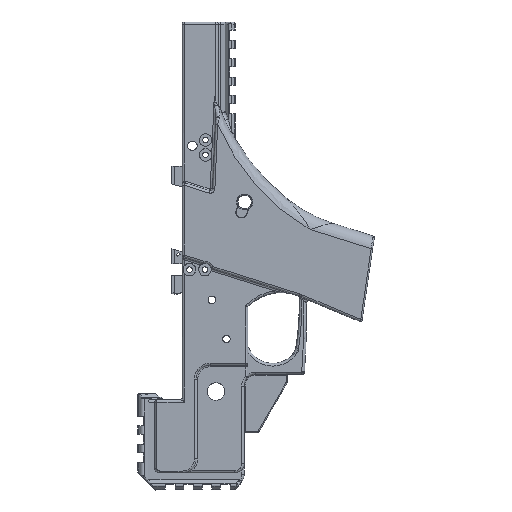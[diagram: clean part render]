
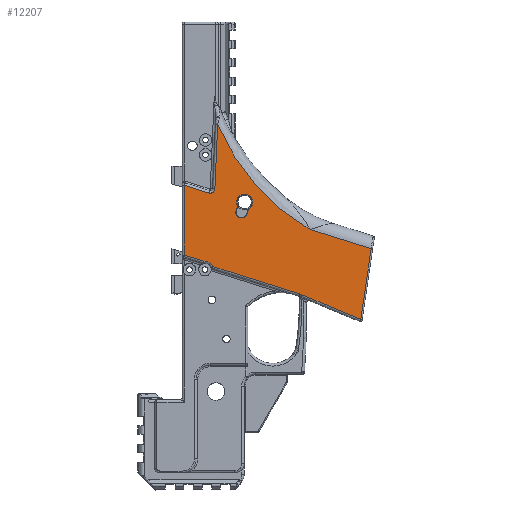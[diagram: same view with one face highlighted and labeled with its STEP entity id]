
A CAD part, left-side view. The second image highlights one B-rep face of the part: STEP entity #12207.
In plain terms, the highlighted planar face has unit normal (-1, 0, 0).
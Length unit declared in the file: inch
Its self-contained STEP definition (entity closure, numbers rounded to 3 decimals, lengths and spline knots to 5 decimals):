
#533=FACE_BOUND('',#3957,.T.);
#667=PLANE('',#13263);
#1186=LINE('',#20847,#2080);
#1207=LINE('',#21066,#2101);
#1209=LINE('',#21087,#2103);
#1211=LINE('',#21092,#2105);
#1212=LINE('',#21096,#2106);
#1213=LINE('',#21098,#2107);
#1214=LINE('',#21100,#2108);
#1215=LINE('',#21104,#2109);
#1216=LINE('',#21108,#2110);
#1217=LINE('',#21112,#2111);
#2080=VECTOR('',#15531,0.3937);
#2101=VECTOR('',#15582,0.3937);
#2103=VECTOR('',#15588,0.3937);
#2105=VECTOR('',#15594,0.3937);
#2106=VECTOR('',#15597,0.3937);
#2107=VECTOR('',#15598,0.3937);
#2108=VECTOR('',#15599,0.3937);
#2109=VECTOR('',#15602,0.3937);
#2110=VECTOR('',#15605,0.3937);
#2111=VECTOR('',#15608,0.3937);
#3211=FACE_OUTER_BOUND('',#3956,.T.);
#3956=EDGE_LOOP('',(#9567,#9568,#9569,#9570,#9571,#9572,#9573,#9574,#9575,
#9576,#9577,#9578));
#3957=EDGE_LOOP('',(#9579,#9580,#9581,#9582));
#4623=CIRCLE('',#13041,4.82183);
#4734=CIRCLE('',#13264,0.1);
#4735=CIRCLE('',#13265,0.1845);
#4736=CIRCLE('',#13266,0.55);
#4737=CIRCLE('',#13267,0.124);
#4738=CIRCLE('',#13268,0.1725);
#5377=VERTEX_POINT('',#19452);
#5378=VERTEX_POINT('',#19458);
#5590=VERTEX_POINT('',#20837);
#5592=VERTEX_POINT('',#20843);
#5626=VERTEX_POINT('',#21065);
#5628=VERTEX_POINT('',#21091);
#5629=VERTEX_POINT('',#21093);
#5630=VERTEX_POINT('',#21095);
#5631=VERTEX_POINT('',#21097);
#5632=VERTEX_POINT('',#21099);
#5633=VERTEX_POINT('',#21101);
#5634=VERTEX_POINT('',#21103);
#5635=VERTEX_POINT('',#21106);
#5636=VERTEX_POINT('',#21107);
#5637=VERTEX_POINT('',#21109);
#5638=VERTEX_POINT('',#21111);
#6702=EDGE_CURVE('',#5378,#5377,#4623,.T.);
#7018=EDGE_CURVE('',#5590,#5592,#1186,.T.);
#7057=EDGE_CURVE('',#5592,#5626,#1207,.T.);
#7061=EDGE_CURVE('',#5378,#5590,#1209,.T.);
#7063=EDGE_CURVE('',#5628,#5377,#1211,.T.);
#7064=EDGE_CURVE('',#5629,#5628,#4734,.T.);
#7065=EDGE_CURVE('',#5630,#5629,#1212,.T.);
#7066=EDGE_CURVE('',#5631,#5630,#1213,.T.);
#7067=EDGE_CURVE('',#5632,#5631,#1214,.T.);
#7068=EDGE_CURVE('',#5633,#5632,#4735,.T.);
#7069=EDGE_CURVE('',#5634,#5633,#1215,.T.);
#7070=EDGE_CURVE('',#5626,#5634,#4736,.T.);
#7071=EDGE_CURVE('',#5635,#5636,#1216,.T.);
#7072=EDGE_CURVE('',#5637,#5635,#4737,.T.);
#7073=EDGE_CURVE('',#5638,#5637,#1217,.T.);
#7074=EDGE_CURVE('',#5636,#5638,#4738,.T.);
#9567=ORIENTED_EDGE('',*,*,#7018,.F.);
#9568=ORIENTED_EDGE('',*,*,#7061,.F.);
#9569=ORIENTED_EDGE('',*,*,#6702,.T.);
#9570=ORIENTED_EDGE('',*,*,#7063,.F.);
#9571=ORIENTED_EDGE('',*,*,#7064,.F.);
#9572=ORIENTED_EDGE('',*,*,#7065,.F.);
#9573=ORIENTED_EDGE('',*,*,#7066,.F.);
#9574=ORIENTED_EDGE('',*,*,#7067,.F.);
#9575=ORIENTED_EDGE('',*,*,#7068,.F.);
#9576=ORIENTED_EDGE('',*,*,#7069,.F.);
#9577=ORIENTED_EDGE('',*,*,#7070,.F.);
#9578=ORIENTED_EDGE('',*,*,#7057,.F.);
#9579=ORIENTED_EDGE('',*,*,#7071,.F.);
#9580=ORIENTED_EDGE('',*,*,#7072,.F.);
#9581=ORIENTED_EDGE('',*,*,#7073,.F.);
#9582=ORIENTED_EDGE('',*,*,#7074,.F.);
#12207=ADVANCED_FACE('',(#3211,#533),#667,.T.);
#13041=AXIS2_PLACEMENT_3D('',#19459,#14977,#14978);
#13263=AXIS2_PLACEMENT_3D('',#21090,#15592,#15593);
#13264=AXIS2_PLACEMENT_3D('',#21094,#15595,#15596);
#13265=AXIS2_PLACEMENT_3D('',#21102,#15600,#15601);
#13266=AXIS2_PLACEMENT_3D('',#21105,#15603,#15604);
#13267=AXIS2_PLACEMENT_3D('',#21110,#15606,#15607);
#13268=AXIS2_PLACEMENT_3D('',#21113,#15609,#15610);
#14977=DIRECTION('center_axis',(1.,0.,0.));
#14978=DIRECTION('ref_axis',(0.,-0.858,0.513));
#15531=DIRECTION('',(0.,0.146,-0.989));
#15582=DIRECTION('',(0.,0.922,0.386));
#15588=DIRECTION('',(0.,-0.954,-0.301));
#15592=DIRECTION('center_axis',(-1.,0.,0.));
#15593=DIRECTION('ref_axis',(0.,0.301,-0.954));
#15594=DIRECTION('',(0.,-0.044,0.999));
#15595=DIRECTION('center_axis',(-1.,0.,0.));
#15596=DIRECTION('ref_axis',(0.,-0.574,-0.819));
#15597=DIRECTION('',(0.,-0.954,-0.301));
#15598=DIRECTION('',(0.,0.,1.));
#15599=DIRECTION('',(0.,0.954,0.301));
#15600=DIRECTION('center_axis',(-1.,0.,0.));
#15601=DIRECTION('ref_axis',(0.,-0.536,0.844));
#15602=DIRECTION('',(0.,0.954,0.301));
#15603=DIRECTION('center_axis',(-1.,0.,0.));
#15604=DIRECTION('ref_axis',(0.,-0.344,0.939));
#15605=DIRECTION('',(0.,-0.301,0.954));
#15606=DIRECTION('center_axis',(-1.,0.,0.));
#15607=DIRECTION('ref_axis',(0.,0.301,-0.954));
#15608=DIRECTION('',(0.,0.301,-0.954));
#15609=DIRECTION('center_axis',(-1.,0.,0.));
#15610=DIRECTION('ref_axis',(0.,-0.301,0.954));
#19452=CARTESIAN_POINT('',(-0.63,-0.54257,0.45432));
#19458=CARTESIAN_POINT('',(-0.63,-2.52341,-1.79711));
#19459=CARTESIAN_POINT('Origin',(-0.63,-4.97366,2.35575));
#20837=CARTESIAN_POINT('',(-0.63,-3.83543,-2.21079));
#20843=CARTESIAN_POINT('',(-0.63,-3.61188,-3.72465));
#20847=CARTESIAN_POINT('',(-0.63,-3.1983,-6.52542));
#21065=CARTESIAN_POINT('',(-0.63,-2.34601,-3.19423));
#21066=CARTESIAN_POINT('',(-0.63,-2.64354,-3.31889));
#21087=CARTESIAN_POINT('',(-0.63,-3.86992,-2.22167));
#21090=CARTESIAN_POINT('Origin',(-0.63,-3.86992,-2.22167));
#21091=CARTESIAN_POINT('',(-0.63,-0.48252,-0.92102));
#21092=CARTESIAN_POINT('',(-0.63,-0.4624,-1.38187));
#21093=CARTESIAN_POINT('',(-0.63,-0.35255,-1.01203));
#21094=CARTESIAN_POINT('Origin',(-0.63,-0.38262,
-0.91666));
#21095=CARTESIAN_POINT('',(-0.63,0.171,-0.84696));
#21096=CARTESIAN_POINT('',(-0.63,-1.83137,-1.4783));
#21097=CARTESIAN_POINT('',(-0.63,0.171,-2.34578));
#21098=CARTESIAN_POINT('',(-0.63,0.171,-0.68592));
#21099=CARTESIAN_POINT('',(-0.63,-0.23911,-2.47509));
#21100=CARTESIAN_POINT('',(-0.63,-1.92231,-3.0058));
#21101=CARTESIAN_POINT('',(-0.63,-0.44101,-2.59117));
#21102=CARTESIAN_POINT('Origin',(-0.63,-0.26873,
-2.6572));
#21103=CARTESIAN_POINT('',(-0.63,-2.29885,-3.17695));
#21104=CARTESIAN_POINT('',(-0.63,-3.45389,-3.54113));
#21105=CARTESIAN_POINT('Origin',(-0.63,-2.13346,-3.70149));
#21106=CARTESIAN_POINT('',(-0.63,-1.17219,-1.46199));
#21107=CARTESIAN_POINT('',(-0.63,-1.20439,-1.35986));
#21108=CARTESIAN_POINT('',(-0.63,-1.21936,-1.31239));
#21109=CARTESIAN_POINT('',(-0.63,-0.93567,-1.38741));
#21110=CARTESIAN_POINT('Origin',(-0.63,-1.05393,-1.4247));
#21111=CARTESIAN_POINT('',(-0.63,-0.96787,-1.28529));
#21112=CARTESIAN_POINT('',(-0.63,-0.9487,-1.34607));
#21113=CARTESIAN_POINT('Origin',(-0.63,-1.12219,-1.20821));
